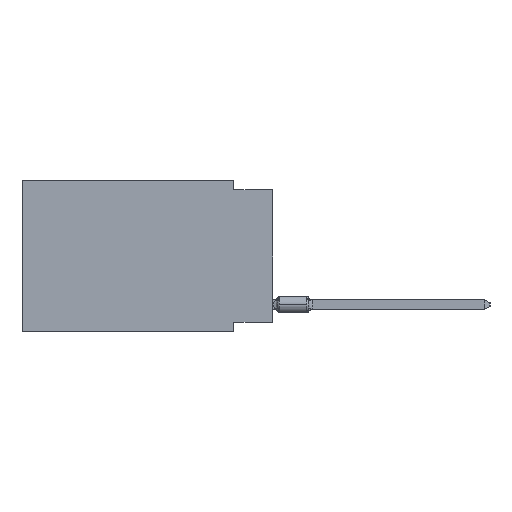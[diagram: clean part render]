
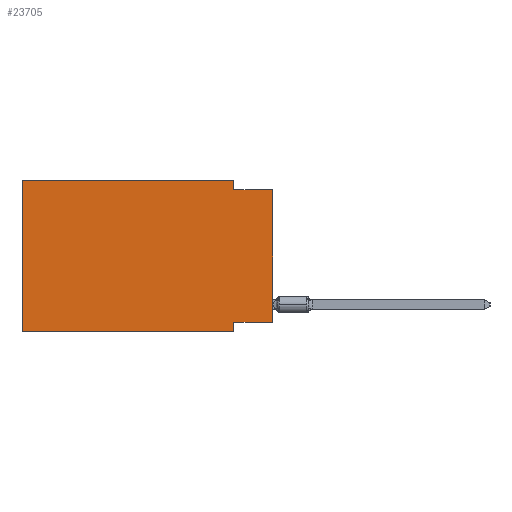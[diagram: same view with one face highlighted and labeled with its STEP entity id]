
A CAD part, left-side view. The second image highlights one B-rep face of the part: STEP entity #23705.
In plain terms, the highlighted planar face has unit normal (-1, 0, 0).
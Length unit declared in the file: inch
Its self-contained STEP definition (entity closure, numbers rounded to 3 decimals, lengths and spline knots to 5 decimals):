
#433 = LINE ( 'NONE', #24694, #27364 ) ;
#564 = CARTESIAN_POINT ( 'NONE',  ( 0., 0.645, 0. ) ) ;
#621 = DIRECTION ( 'NONE',  ( 0., 0., -1. ) ) ;
#720 = ORIENTED_EDGE ( 'NONE', *, *, #12084, .F. ) ;
#1852 = LINE ( 'NONE', #11696, #29156 ) ;
#2004 = EDGE_CURVE ( 'NONE', #7769, #19667, #1852, .T. ) ;
#2237 = VERTEX_POINT ( 'NONE', #19682 ) ;
#2918 = LINE ( 'NONE', #15171, #6085 ) ;
#3145 = EDGE_CURVE ( 'NONE', #11828, #9284, #9416, .T. ) ;
#4325 = EDGE_CURVE ( 'NONE', #29130, #2237, #9124, .T. ) ;
#4468 = VECTOR ( 'NONE', #27071, 39.37008 ) ;
#4581 = DIRECTION ( 'NONE',  ( 0., 1., 0. ) ) ;
#5018 = CARTESIAN_POINT ( 'NONE',  ( 0., 0.1, 0. ) ) ;
#5304 = PLANE ( 'NONE',  #31624 ) ;
#5423 = DIRECTION ( 'NONE',  ( 0., 0., 1. ) ) ;
#5626 = CARTESIAN_POINT ( 'NONE',  ( 0., 0.645, 0. ) ) ;
#6085 = VECTOR ( 'NONE', #17448, 39.37008 ) ;
#6560 = EDGE_CURVE ( 'NONE', #21703, #2237, #2918, .T. ) ;
#7769 = VERTEX_POINT ( 'NONE', #12593 ) ;
#7791 = ORIENTED_EDGE ( 'NONE', *, *, #6560, .T. ) ;
#9124 = LINE ( 'NONE', #29191, #4468 ) ;
#9284 = VERTEX_POINT ( 'NONE', #26816 ) ;
#9416 = LINE ( 'NONE', #14117, #15124 ) ;
#10636 = DIRECTION ( 'NONE',  ( 1., 0., 0. ) ) ;
#11696 = CARTESIAN_POINT ( 'NONE',  ( 0., 0., 0. ) ) ;
#11828 = VERTEX_POINT ( 'NONE', #5018 ) ;
#12084 = EDGE_CURVE ( 'NONE', #9284, #19667, #12207, .T. ) ;
#12207 = LINE ( 'NONE', #19637, #30724 ) ;
#12593 = CARTESIAN_POINT ( 'NONE',  ( 0., 0., -0.365 ) ) ;
#12677 = ORIENTED_EDGE ( 'NONE', *, *, #4325, .F. ) ;
#13062 = VERTEX_POINT ( 'NONE', #5626 ) ;
#14117 = CARTESIAN_POINT ( 'NONE',  ( 0., 0.1, 0. ) ) ;
#15124 = VECTOR ( 'NONE', #23988, 39.37008 ) ;
#15171 = CARTESIAN_POINT ( 'NONE',  ( 0., 0.645, -0.39 ) ) ;
#16753 = ORIENTED_EDGE ( 'NONE', *, *, #20146, .F. ) ;
#17093 = ORIENTED_EDGE ( 'NONE', *, *, #2004, .T. ) ;
#17274 = EDGE_CURVE ( 'NONE', #21703, #13062, #24992, .T. ) ;
#17287 = ORIENTED_EDGE ( 'NONE', *, *, #30662, .F. ) ;
#17448 = DIRECTION ( 'NONE',  ( 0., -1., 0. ) ) ;
#17978 = CARTESIAN_POINT ( 'NONE',  ( 0., 0.645, -0.39 ) ) ;
#19637 = CARTESIAN_POINT ( 'NONE',  ( 0., 0., -0.025 ) ) ;
#19667 = VERTEX_POINT ( 'NONE', #25217 ) ;
#19682 = CARTESIAN_POINT ( 'NONE',  ( 0., 0.1, -0.39 ) ) ;
#20102 = CARTESIAN_POINT ( 'NONE',  ( 0., 0.1, -0.365 ) ) ;
#20136 = DIRECTION ( 'NONE',  ( 0., -1., 0. ) ) ;
#20146 = EDGE_CURVE ( 'NONE', #13062, #11828, #433, .T. ) ;
#20845 = EDGE_LOOP ( 'NONE', ( #17093, #720, #31438, #16753, #21051, #7791, #12677, #17287 ) ) ;
#21051 = ORIENTED_EDGE ( 'NONE', *, *, #17274, .F. ) ;
#21568 = DIRECTION ( 'NONE',  ( 0., 0., 1. ) ) ;
#21703 = VERTEX_POINT ( 'NONE', #17978 ) ;
#22771 = CARTESIAN_POINT ( 'NONE',  ( 0., 0.645, 0. ) ) ;
#23705 = ADVANCED_FACE ( 'NONE', ( #25221 ), #5304, .F. ) ;
#23988 = DIRECTION ( 'NONE',  ( 0., 0., -1. ) ) ;
#24187 = DIRECTION ( 'NONE',  ( 0., -1., 0. ) ) ;
#24694 = CARTESIAN_POINT ( 'NONE',  ( 0., 0.645, 0. ) ) ;
#24992 = LINE ( 'NONE', #564, #29339 ) ;
#25217 = CARTESIAN_POINT ( 'NONE',  ( 0., 0., -0.025 ) ) ;
#25221 = FACE_OUTER_BOUND ( 'NONE', #20845, .T. ) ;
#26735 = LINE ( 'NONE', #26884, #31791 ) ;
#26816 = CARTESIAN_POINT ( 'NONE',  ( 0., 0.1, -0.025 ) ) ;
#26884 = CARTESIAN_POINT ( 'NONE',  ( 0., 0., -0.365 ) ) ;
#27071 = DIRECTION ( 'NONE',  ( 0., 0., -1. ) ) ;
#27364 = VECTOR ( 'NONE', #20136, 39.37008 ) ;
#29130 = VERTEX_POINT ( 'NONE', #20102 ) ;
#29156 = VECTOR ( 'NONE', #21568, 39.37008 ) ;
#29191 = CARTESIAN_POINT ( 'NONE',  ( 0., 0.1, -0.39 ) ) ;
#29339 = VECTOR ( 'NONE', #5423, 39.37008 ) ;
#30662 = EDGE_CURVE ( 'NONE', #7769, #29130, #26735, .T. ) ;
#30724 = VECTOR ( 'NONE', #24187, 39.37008 ) ;
#31438 = ORIENTED_EDGE ( 'NONE', *, *, #3145, .F. ) ;
#31624 = AXIS2_PLACEMENT_3D ( 'NONE', #22771, #10636, #621 ) ;
#31791 = VECTOR ( 'NONE', #4581, 39.37008 ) ;
